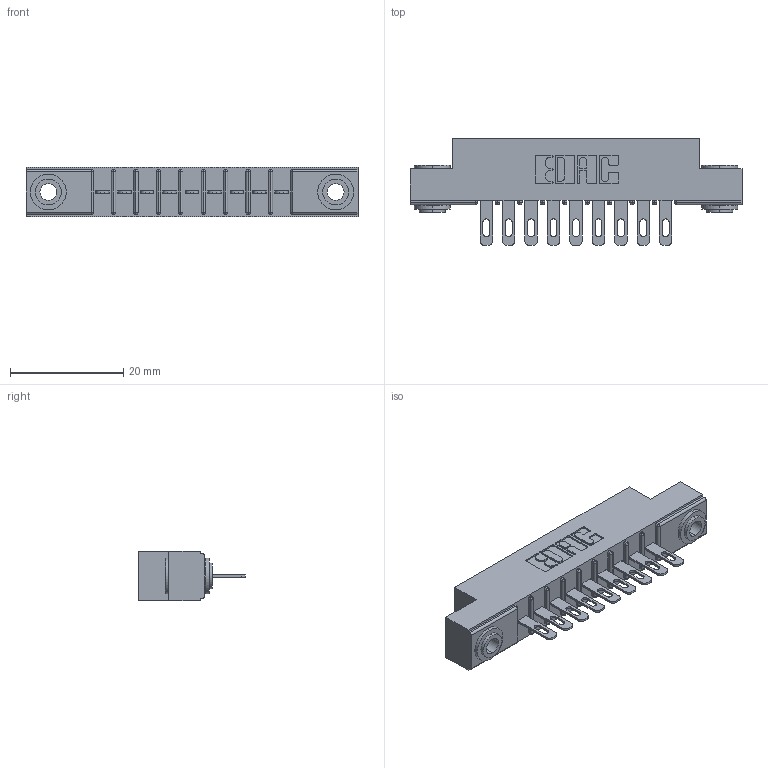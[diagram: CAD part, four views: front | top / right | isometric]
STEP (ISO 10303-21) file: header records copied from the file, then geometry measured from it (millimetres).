
FILE_DESCRIPTION (( 'STEP AP203' ), '1' );
FILE_NAME ('316-009-500-103.STEP', '2018-07-30T23:56:52', ( '' ), ( '' ), 'SwSTEP 2.0', 'SolidWorks 2016', '' );
FILE_SCHEMA (( 'CONFIG_CONTROL_DESIGN' ));
Length unit declared in the file: inch
Products named in the file (4): 306 Part_.156 Dia; 306-290-001_100; 345-250-002_345-250-002-102; 316-009-500-103
Assembly tree (12 placements, depth 2):
  316-009-500-103
    306 Part_.156 Dia
    306-290-001_100  x9
    345-250-002_345-250-002-102  x2
Bounding box: 58.67 x 18.87 x 8.71 mm (x, y, z)
Volume: 3989.7 mm3; surface area: 5875.8 mm2
Topology: 12 solids, 12 shells, 852 faces, 2363 edges, 1522 vertices
Faces by surface type: plane 542, cylinder 266, sphere 36, cone 8
Entity records: 13897 total; most frequent: CARTESIAN_POINT 2307, DIRECTION 2293, ORIENTED_EDGE 2274, EDGE_CURVE 1137, LINE 861, VECTOR 861, VERTEX_POINT 730, AXIS2_PLACEMENT_3D 716
